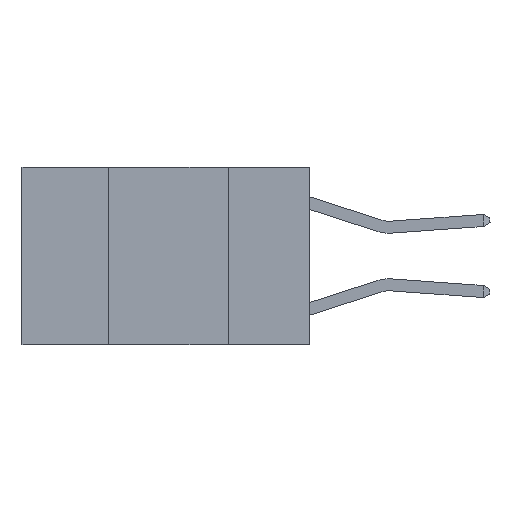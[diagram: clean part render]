
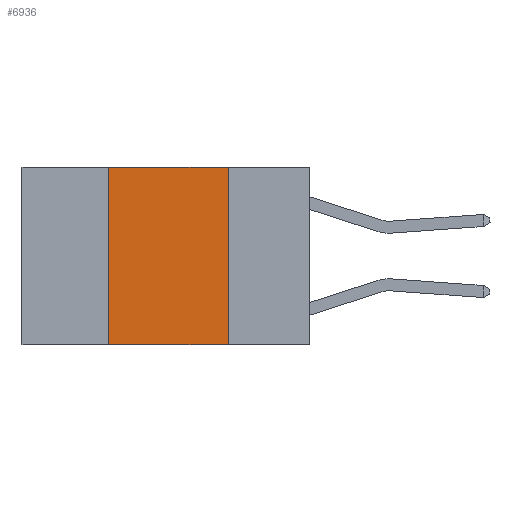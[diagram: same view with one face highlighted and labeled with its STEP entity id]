
A CAD part, left-side view. The second image highlights one B-rep face of the part: STEP entity #6936.
In plain terms, the highlighted planar face has unit normal (-1, 0, 0).
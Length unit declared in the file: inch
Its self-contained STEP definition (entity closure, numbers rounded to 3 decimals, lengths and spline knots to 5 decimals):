
#47 = LINE ( 'NONE', #1978, #24574 ) ;
#342 = VECTOR ( 'NONE', #18764, 39.37008 ) ;
#916 = CARTESIAN_POINT ( 'NONE',  ( 0., 0.42, -0.37 ) ) ;
#1819 = FACE_OUTER_BOUND ( 'NONE', #20769, .T. ) ;
#1978 = CARTESIAN_POINT ( 'NONE',  ( 0., 0.6, -0.37 ) ) ;
#2018 = CARTESIAN_POINT ( 'NONE',  ( 0., 0.17, 0. ) ) ;
#2278 = ORIENTED_EDGE ( 'NONE', *, *, #9236, .F. ) ;
#2942 = VERTEX_POINT ( 'NONE', #2018 ) ;
#3353 = VERTEX_POINT ( 'NONE', #22830 ) ;
#4314 = DIRECTION ( 'NONE',  ( 0., -1., 0. ) ) ;
#4778 = VECTOR ( 'NONE', #8523, 39.37008 ) ;
#5277 = CARTESIAN_POINT ( 'NONE',  ( 0., 0.17, 0. ) ) ;
#5872 = DIRECTION ( 'NONE',  ( 0., -1., 0. ) ) ;
#6442 = LINE ( 'NONE', #15752, #7068 ) ;
#6573 = ORIENTED_EDGE ( 'NONE', *, *, #15353, .F. ) ;
#6936 = ADVANCED_FACE ( 'NONE', ( #1819 ), #15149, .F. ) ;
#7068 = VECTOR ( 'NONE', #4314, 39.37008 ) ;
#8257 = CARTESIAN_POINT ( 'NONE',  ( 0., 0.42, 0. ) ) ;
#8523 = DIRECTION ( 'NONE',  ( 0., 0., 1. ) ) ;
#9236 = EDGE_CURVE ( 'NONE', #12954, #3353, #22042, .T. ) ;
#11242 = DIRECTION ( 'NONE',  ( 1., 0., 0. ) ) ;
#12727 = ORIENTED_EDGE ( 'NONE', *, *, #13363, .F. ) ;
#12954 = VERTEX_POINT ( 'NONE', #916 ) ;
#13162 = AXIS2_PLACEMENT_3D ( 'NONE', #19193, #11242, #14899 ) ;
#13363 = EDGE_CURVE ( 'NONE', #3353, #2942, #6442, .T. ) ;
#14899 = DIRECTION ( 'NONE',  ( 0., 0., -1. ) ) ;
#15149 = PLANE ( 'NONE',  #13162 ) ;
#15305 = VERTEX_POINT ( 'NONE', #21578 ) ;
#15353 = EDGE_CURVE ( 'NONE', #2942, #15305, #16482, .T. ) ;
#15752 = CARTESIAN_POINT ( 'NONE',  ( 0., 0.6, 0. ) ) ;
#16482 = LINE ( 'NONE', #5277, #342 ) ;
#18764 = DIRECTION ( 'NONE',  ( 0., 0., -1. ) ) ;
#19193 = CARTESIAN_POINT ( 'NONE',  ( 0., 0.6, 0. ) ) ;
#20769 = EDGE_LOOP ( 'NONE', ( #6573, #12727, #2278, #22562 ) ) ;
#21189 = EDGE_CURVE ( 'NONE', #12954, #15305, #47, .T. ) ;
#21578 = CARTESIAN_POINT ( 'NONE',  ( 0., 0.17, -0.37 ) ) ;
#22042 = LINE ( 'NONE', #8257, #4778 ) ;
#22562 = ORIENTED_EDGE ( 'NONE', *, *, #21189, .T. ) ;
#22830 = CARTESIAN_POINT ( 'NONE',  ( 0., 0.42, 0. ) ) ;
#24574 = VECTOR ( 'NONE', #5872, 39.37008 ) ;
